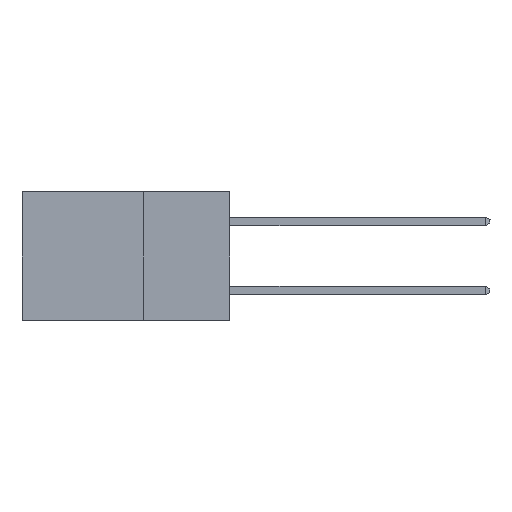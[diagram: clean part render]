
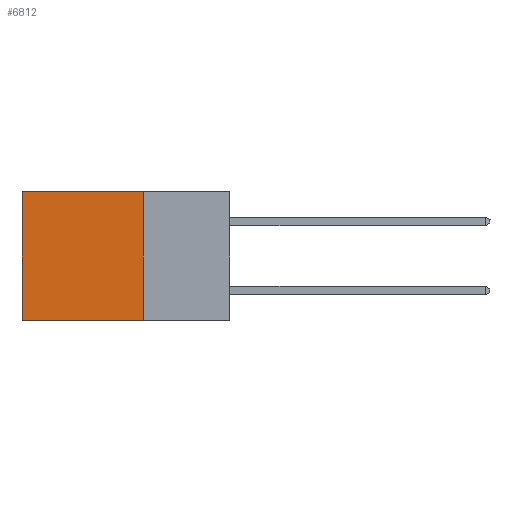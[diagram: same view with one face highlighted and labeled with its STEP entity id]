
A CAD part, left-side view. The second image highlights one B-rep face of the part: STEP entity #6812.
In plain terms, the highlighted planar face has unit normal (-1, 0, 0).
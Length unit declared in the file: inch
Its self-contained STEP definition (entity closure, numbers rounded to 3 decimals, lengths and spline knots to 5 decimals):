
#133 = VERTEX_POINT ( 'NONE', #4177 ) ;
#372 = VERTEX_POINT ( 'NONE', #3972 ) ;
#563 = VECTOR ( 'NONE', #6163, 39.37008 ) ;
#659 = DIRECTION ( 'NONE',  ( 0., 0., -1. ) ) ;
#1318 = DIRECTION ( 'NONE',  ( 0., 0., -1. ) ) ;
#1477 = CARTESIAN_POINT ( 'NONE',  ( 0.2615, 0.25, 0. ) ) ;
#1906 = ORIENTED_EDGE ( 'NONE', *, *, #7074, .F. ) ;
#2608 = ORIENTED_EDGE ( 'NONE', *, *, #11237, .T. ) ;
#2929 = LINE ( 'NONE', #1477, #10801 ) ;
#3022 = EDGE_LOOP ( 'NONE', ( #2608, #5629, #1906, #3325 ) ) ;
#3325 = ORIENTED_EDGE ( 'NONE', *, *, #3576, .T. ) ;
#3438 = DIRECTION ( 'NONE',  ( 1., 0., 0. ) ) ;
#3576 = EDGE_CURVE ( 'NONE', #9856, #10120, #2929, .T. ) ;
#3715 = EDGE_CURVE ( 'NONE', #133, #372, #8031, .T. ) ;
#3972 = CARTESIAN_POINT ( 'NONE',  ( 0.2615, 0.6, -0.37 ) ) ;
#4177 = CARTESIAN_POINT ( 'NONE',  ( 0.2615, 0.25, -0.37 ) ) ;
#5253 = CARTESIAN_POINT ( 'NONE',  ( 0.2615, 0.25, -0.37 ) ) ;
#5629 = ORIENTED_EDGE ( 'NONE', *, *, #3715, .F. ) ;
#5790 = DIRECTION ( 'NONE',  ( 0., 1., 0. ) ) ;
#6106 = PLANE ( 'NONE',  #10003 ) ;
#6163 = DIRECTION ( 'NONE',  ( 0., 0., -1. ) ) ;
#6179 = DIRECTION ( 'NONE',  ( 0., 1., 0. ) ) ;
#6812 = ADVANCED_FACE ( 'NONE', ( #7715 ), #6106, .F. ) ;
#6993 = LINE ( 'NONE', #9876, #563 ) ;
#7074 = EDGE_CURVE ( 'NONE', #9856, #133, #6993, .T. ) ;
#7570 = VECTOR ( 'NONE', #1318, 39.37008 ) ;
#7715 = FACE_OUTER_BOUND ( 'NONE', #3022, .T. ) ;
#8031 = LINE ( 'NONE', #8629, #10976 ) ;
#8629 = CARTESIAN_POINT ( 'NONE',  ( 0.2615, 0.25, -0.37 ) ) ;
#8663 = CARTESIAN_POINT ( 'NONE',  ( 0.2615, 0.25, 0. ) ) ;
#9368 = LINE ( 'NONE', #10318, #7570 ) ;
#9856 = VERTEX_POINT ( 'NONE', #8663 ) ;
#9876 = CARTESIAN_POINT ( 'NONE',  ( 0.2615, 0.25, -0.37 ) ) ;
#10003 = AXIS2_PLACEMENT_3D ( 'NONE', #5253, #3438, #659 ) ;
#10120 = VERTEX_POINT ( 'NONE', #11366 ) ;
#10318 = CARTESIAN_POINT ( 'NONE',  ( 0.2615, 0.6, -0.37 ) ) ;
#10801 = VECTOR ( 'NONE', #5790, 39.37008 ) ;
#10976 = VECTOR ( 'NONE', #6179, 39.37008 ) ;
#11237 = EDGE_CURVE ( 'NONE', #10120, #372, #9368, .T. ) ;
#11366 = CARTESIAN_POINT ( 'NONE',  ( 0.2615, 0.6, 0. ) ) ;
